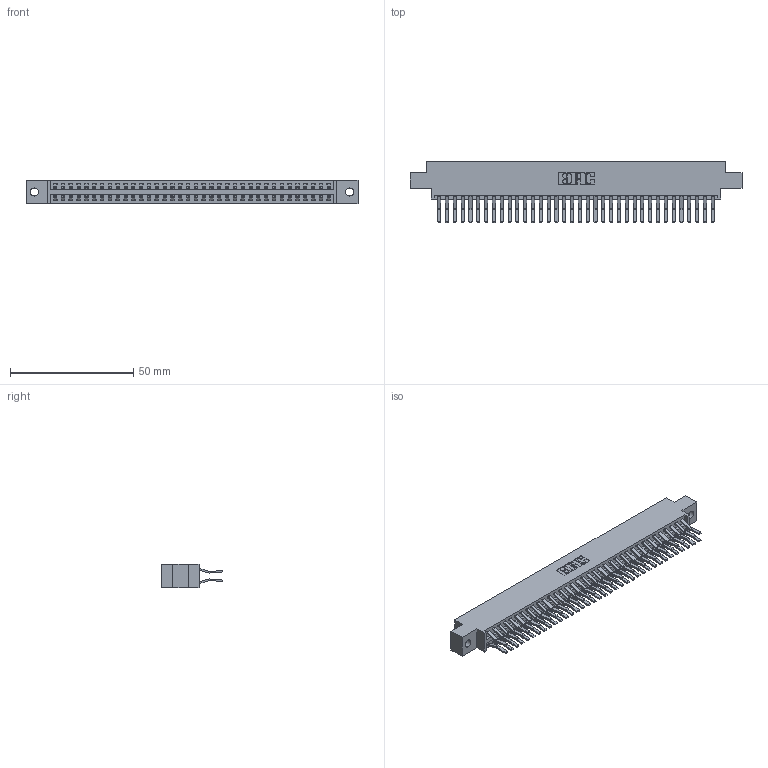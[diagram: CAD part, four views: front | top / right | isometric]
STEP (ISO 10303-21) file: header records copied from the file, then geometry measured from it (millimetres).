
FILE_DESCRIPTION (( 'STEP AP203' ), '1' );
FILE_NAME ('396-072-560-802.STEP', '2019-11-02T11:22:51', ( '' ), ( '' ), 'SwSTEP 2.0', 'SolidWorks 2016', '' );
FILE_SCHEMA (( 'CONFIG_CONTROL_DESIGN' ));
Length unit declared in the file: inch
Products named in the file (3): 346 Part_0.170 Offset - 0.128 Dia; 345-292-001_560 Tail; 396-072-560-802
Assembly tree (73 placements, depth 2):
  396-072-560-802
    346 Part_0.170 Offset - 0.128 Dia
    345-292-001_560 Tail  x72
Bounding box: 134.87 x 24.78 x 9.4 mm (x, y, z)
Volume: 13385.9 mm3; surface area: 19475 mm2
Topology: 73 solids, 73 shells, 4014 faces, 11933 edges, 7858 vertices
Faces by surface type: plane 2600, cylinder 1414
Entity records: 24525 total; most frequent: CARTESIAN_POINT 4052, ORIENTED_EDGE 3986, DIRECTION 3625, EDGE_CURVE 1993, VECTOR 1713, LINE 1713, VERTEX_POINT 1326, AXIS2_PLACEMENT_3D 956
